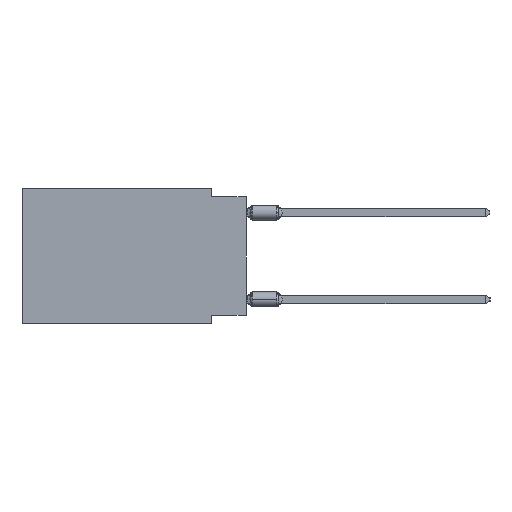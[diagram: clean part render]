
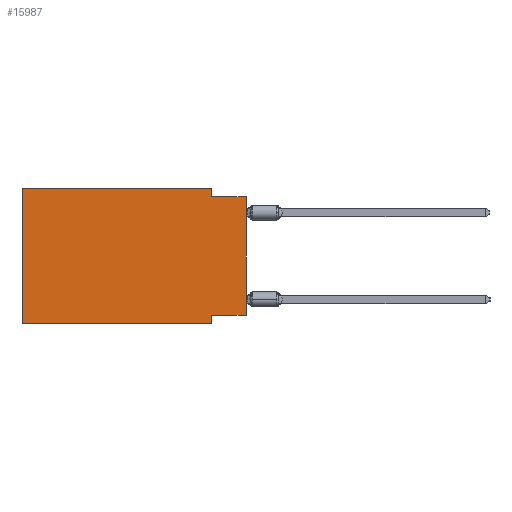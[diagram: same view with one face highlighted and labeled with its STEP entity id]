
A CAD part, left-side view. The second image highlights one B-rep face of the part: STEP entity #15987.
In plain terms, the highlighted planar face has unit normal (-1, 0, 0).
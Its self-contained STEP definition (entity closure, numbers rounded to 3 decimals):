
#138 = VECTOR ( 'NONE', #18558, 1000. ) ;
#606 = FACE_OUTER_BOUND ( 'NONE', #16919, .T. ) ;
#797 = CARTESIAN_POINT ( 'NONE',  ( 0., 16.383, 0. ) ) ;
#899 = AXIS2_PLACEMENT_3D ( 'NONE', #32472, #6399, #27067 ) ;
#4549 = CARTESIAN_POINT ( 'NONE',  ( 0., 0., 0. ) ) ;
#4721 = CARTESIAN_POINT ( 'NONE',  ( 0., 0., -9.271 ) ) ;
#5237 = VECTOR ( 'NONE', #37401, 1000. ) ;
#5254 = CARTESIAN_POINT ( 'NONE',  ( 0., 0., -9.271 ) ) ;
#6399 = DIRECTION ( 'NONE',  ( 1., 0., 0. ) ) ;
#6599 = LINE ( 'NONE', #33054, #138 ) ;
#6696 = VERTEX_POINT ( 'NONE', #7004 ) ;
#6927 = EDGE_CURVE ( 'NONE', #26237, #23334, #37718, .T. ) ;
#7004 = CARTESIAN_POINT ( 'NONE',  ( 0., 16.383, -9.906 ) ) ;
#8587 = EDGE_CURVE ( 'NONE', #6696, #16137, #37341, .T. ) ;
#8696 = EDGE_CURVE ( 'NONE', #6696, #23723, #14704, .T. ) ;
#9761 = VECTOR ( 'NONE', #24635, 1000. ) ;
#9945 = CARTESIAN_POINT ( 'NONE',  ( 0., 0., -0.635 ) ) ;
#10417 = ORIENTED_EDGE ( 'NONE', *, *, #11054, .T. ) ;
#10421 = VECTOR ( 'NONE', #21475, 1000. ) ;
#11054 = EDGE_CURVE ( 'NONE', #26237, #32345, #22712, .T. ) ;
#13528 = CARTESIAN_POINT ( 'NONE',  ( 0., 2.54, -9.271 ) ) ;
#14315 = CARTESIAN_POINT ( 'NONE',  ( 0., 16.383, -9.906 ) ) ;
#14704 = LINE ( 'NONE', #797, #10421 ) ;
#15359 = LINE ( 'NONE', #9945, #9761 ) ;
#15416 = VERTEX_POINT ( 'NONE', #22159 ) ;
#15442 = ORIENTED_EDGE ( 'NONE', *, *, #20647, .F. ) ;
#15987 = ADVANCED_FACE ( 'NONE', ( #606 ), #26671, .F. ) ;
#16137 = VERTEX_POINT ( 'NONE', #24558 ) ;
#16822 = DIRECTION ( 'NONE',  ( 0., 1., 0. ) ) ;
#16919 = EDGE_LOOP ( 'NONE', ( #10417, #32544, #15442, #29566, #27355, #28868, #22394, #31392 ) ) ;
#17910 = DIRECTION ( 'NONE',  ( 0., 0., -1. ) ) ;
#18164 = VECTOR ( 'NONE', #31061, 1000. ) ;
#18558 = DIRECTION ( 'NONE',  ( 0., -1., 0. ) ) ;
#20647 = EDGE_CURVE ( 'NONE', #36887, #15416, #28176, .T. ) ;
#21475 = DIRECTION ( 'NONE',  ( 0., 0., 1. ) ) ;
#21770 = CARTESIAN_POINT ( 'NONE',  ( 0., 2.54, 0. ) ) ;
#22159 = CARTESIAN_POINT ( 'NONE',  ( 0., 2.54, -0.635 ) ) ;
#22394 = ORIENTED_EDGE ( 'NONE', *, *, #29772, .F. ) ;
#22712 = LINE ( 'NONE', #4549, #5237 ) ;
#23334 = VERTEX_POINT ( 'NONE', #13528 ) ;
#23723 = VERTEX_POINT ( 'NONE', #37420 ) ;
#24526 = CARTESIAN_POINT ( 'NONE',  ( 0., 2.54, -9.906 ) ) ;
#24558 = CARTESIAN_POINT ( 'NONE',  ( 0., 2.54, -9.906 ) ) ;
#24635 = DIRECTION ( 'NONE',  ( 0., -1., 0. ) ) ;
#25166 = EDGE_CURVE ( 'NONE', #15416, #32345, #15359, .T. ) ;
#26120 = DIRECTION ( 'NONE',  ( 0., -1., 0. ) ) ;
#26237 = VERTEX_POINT ( 'NONE', #4721 ) ;
#26671 = PLANE ( 'NONE',  #899 ) ;
#26990 = CARTESIAN_POINT ( 'NONE',  ( 0., 2.54, 0. ) ) ;
#27067 = DIRECTION ( 'NONE',  ( 0., 0., -1. ) ) ;
#27355 = ORIENTED_EDGE ( 'NONE', *, *, #8696, .F. ) ;
#28176 = LINE ( 'NONE', #26990, #32122 ) ;
#28868 = ORIENTED_EDGE ( 'NONE', *, *, #8587, .T. ) ;
#29566 = ORIENTED_EDGE ( 'NONE', *, *, #31812, .F. ) ;
#29772 = EDGE_CURVE ( 'NONE', #23334, #16137, #33784, .T. ) ;
#30663 = VECTOR ( 'NONE', #16822, 1000. ) ;
#30801 = VECTOR ( 'NONE', #26120, 1000. ) ;
#31061 = DIRECTION ( 'NONE',  ( 0., 0., -1. ) ) ;
#31392 = ORIENTED_EDGE ( 'NONE', *, *, #6927, .F. ) ;
#31812 = EDGE_CURVE ( 'NONE', #23723, #36887, #6599, .T. ) ;
#32122 = VECTOR ( 'NONE', #17910, 1000. ) ;
#32345 = VERTEX_POINT ( 'NONE', #37234 ) ;
#32472 = CARTESIAN_POINT ( 'NONE',  ( 0., 16.383, 0. ) ) ;
#32544 = ORIENTED_EDGE ( 'NONE', *, *, #25166, .F. ) ;
#33054 = CARTESIAN_POINT ( 'NONE',  ( 0., 16.383, 0. ) ) ;
#33784 = LINE ( 'NONE', #24526, #18164 ) ;
#36887 = VERTEX_POINT ( 'NONE', #21770 ) ;
#37234 = CARTESIAN_POINT ( 'NONE',  ( 0., 0., -0.635 ) ) ;
#37341 = LINE ( 'NONE', #14315, #30801 ) ;
#37401 = DIRECTION ( 'NONE',  ( 0., 0., 1. ) ) ;
#37420 = CARTESIAN_POINT ( 'NONE',  ( 0., 16.383, 0. ) ) ;
#37718 = LINE ( 'NONE', #5254, #30663 ) ;
